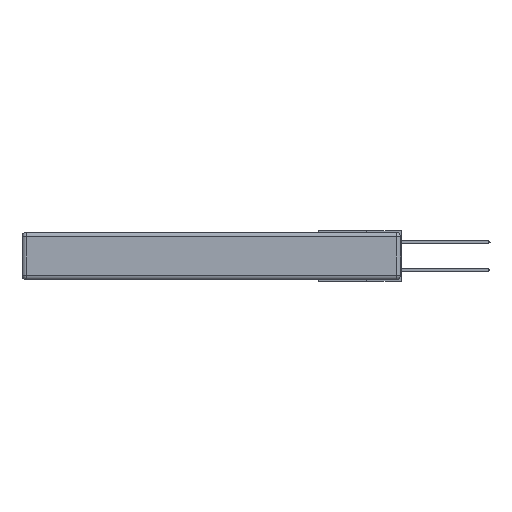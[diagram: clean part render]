
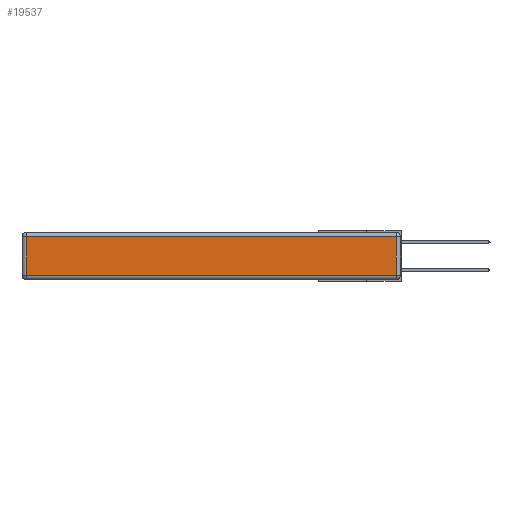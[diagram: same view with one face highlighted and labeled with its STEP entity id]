
A CAD part, left-side view. The second image highlights one B-rep face of the part: STEP entity #19537.
In plain terms, the highlighted planar face has unit normal (-1, 0, 0).
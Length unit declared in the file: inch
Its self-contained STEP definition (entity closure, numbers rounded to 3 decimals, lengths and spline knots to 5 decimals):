
#342 = LINE ( 'NONE', #16489, #4850 ) ;
#1127 = EDGE_CURVE ( 'NONE', #22676, #10779, #15326, .T. ) ;
#1718 = DIRECTION ( 'NONE',  ( 0., 0., 1. ) ) ;
#3079 = DIRECTION ( 'NONE',  ( 0., 0., -1. ) ) ;
#4850 = VECTOR ( 'NONE', #3079, 39.37008 ) ;
#7684 = LINE ( 'NONE', #29091, #21678 ) ;
#8748 = DIRECTION ( 'NONE',  ( 0., 1., 0. ) ) ;
#10200 = CARTESIAN_POINT ( 'NONE',  ( 0., 2.72, -0.03 ) ) ;
#10779 = VERTEX_POINT ( 'NONE', #10200 ) ;
#11489 = CARTESIAN_POINT ( 'NONE',  ( 0., 2.75, -0.03 ) ) ;
#12693 = AXIS2_PLACEMENT_3D ( 'NONE', #33134, #22825, #1718 ) ;
#15326 = LINE ( 'NONE', #11489, #32704 ) ;
#15668 = FACE_OUTER_BOUND ( 'NONE', #33493, .T. ) ;
#16489 = CARTESIAN_POINT ( 'NONE',  ( 0., 2.72, -0.343 ) ) ;
#16568 = DIRECTION ( 'NONE',  ( 0., -1., 0. ) ) ;
#19537 = ADVANCED_FACE ( 'NONE', ( #15668 ), #20184, .T. ) ;
#19762 = ORIENTED_EDGE ( 'NONE', *, *, #28638, .T. ) ;
#20184 = PLANE ( 'NONE',  #12693 ) ;
#20814 = ORIENTED_EDGE ( 'NONE', *, *, #33474, .T. ) ;
#20845 = VECTOR ( 'NONE', #16568, 39.37008 ) ;
#21265 = VERTEX_POINT ( 'NONE', #29664 ) ;
#21678 = VECTOR ( 'NONE', #31616, 39.37008 ) ;
#22676 = VERTEX_POINT ( 'NONE', #29343 ) ;
#22825 = DIRECTION ( 'NONE',  ( -1., 0., 0. ) ) ;
#22943 = ORIENTED_EDGE ( 'NONE', *, *, #33763, .T. ) ;
#27894 = LINE ( 'NONE', #29841, #20845 ) ;
#28638 = EDGE_CURVE ( 'NONE', #29617, #22676, #7684, .T. ) ;
#29091 = CARTESIAN_POINT ( 'NONE',  ( 0., 0.03, -0.343 ) ) ;
#29165 = ORIENTED_EDGE ( 'NONE', *, *, #1127, .T. ) ;
#29343 = CARTESIAN_POINT ( 'NONE',  ( 0., 0.03, -0.03 ) ) ;
#29617 = VERTEX_POINT ( 'NONE', #31874 ) ;
#29664 = CARTESIAN_POINT ( 'NONE',  ( 0., 2.72, -0.313 ) ) ;
#29841 = CARTESIAN_POINT ( 'NONE',  ( 0., 0., -0.313 ) ) ;
#31616 = DIRECTION ( 'NONE',  ( 0., 0., 1. ) ) ;
#31874 = CARTESIAN_POINT ( 'NONE',  ( 0., 0.03, -0.313 ) ) ;
#32704 = VECTOR ( 'NONE', #8748, 39.37008 ) ;
#33134 = CARTESIAN_POINT ( 'NONE',  ( 0., 0., -0.343 ) ) ;
#33474 = EDGE_CURVE ( 'NONE', #10779, #21265, #342, .T. ) ;
#33493 = EDGE_LOOP ( 'NONE', ( #22943, #19762, #29165, #20814 ) ) ;
#33763 = EDGE_CURVE ( 'NONE', #21265, #29617, #27894, .T. ) ;
